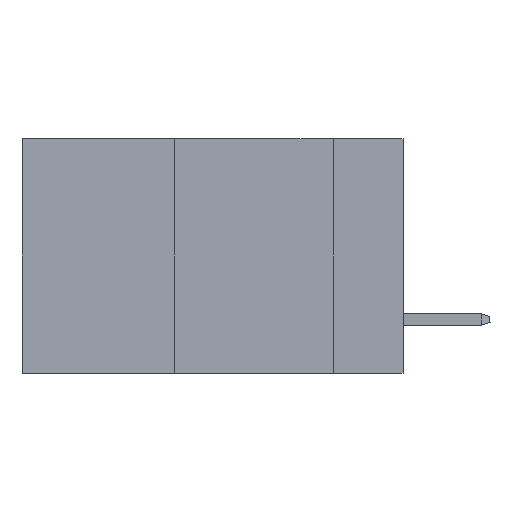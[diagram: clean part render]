
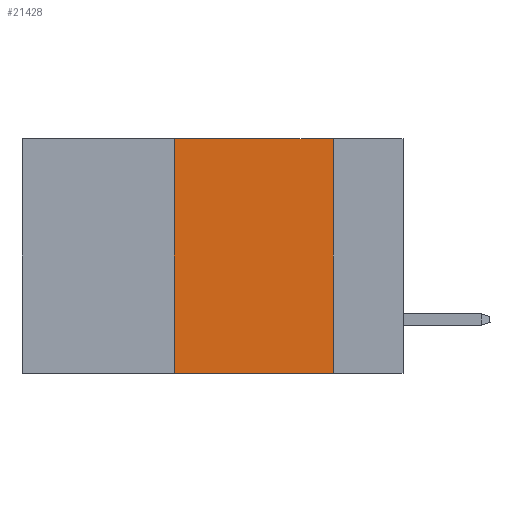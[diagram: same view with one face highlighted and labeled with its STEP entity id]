
A CAD part, left-side view. The second image highlights one B-rep face of the part: STEP entity #21428.
In plain terms, the highlighted planar face has unit normal (-1, 0, 0).
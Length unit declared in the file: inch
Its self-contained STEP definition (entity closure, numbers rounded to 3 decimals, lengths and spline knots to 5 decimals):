
#226 = CARTESIAN_POINT ( 'NONE',  ( 0., 0.11, -0.37 ) ) ;
#608 = VECTOR ( 'NONE', #22366, 39.37008 ) ;
#1459 = DIRECTION ( 'NONE',  ( 0., 0., -1. ) ) ;
#1627 = VECTOR ( 'NONE', #17815, 39.37008 ) ;
#2300 = DIRECTION ( 'NONE',  ( 0., 0., -1. ) ) ;
#2961 = CARTESIAN_POINT ( 'NONE',  ( 0., 0.11, 0. ) ) ;
#3543 = EDGE_CURVE ( 'NONE', #16228, #36907, #26728, .T. ) ;
#8606 = VERTEX_POINT ( 'NONE', #15901 ) ;
#11014 = EDGE_CURVE ( 'NONE', #8606, #16228, #23114, .T. ) ;
#11662 = DIRECTION ( 'NONE',  ( 0., -1., 0. ) ) ;
#12409 = EDGE_LOOP ( 'NONE', ( #28049, #28809, #15225, #15103 ) ) ;
#13007 = CARTESIAN_POINT ( 'NONE',  ( 0., 0.11, 0. ) ) ;
#13609 = CARTESIAN_POINT ( 'NONE',  ( 0., 0.36, 0. ) ) ;
#15103 = ORIENTED_EDGE ( 'NONE', *, *, #16697, .T. ) ;
#15225 = ORIENTED_EDGE ( 'NONE', *, *, #11014, .F. ) ;
#15299 = LINE ( 'NONE', #13007, #22468 ) ;
#15901 = CARTESIAN_POINT ( 'NONE',  ( 0., 0.36, -0.37 ) ) ;
#15935 = AXIS2_PLACEMENT_3D ( 'NONE', #28811, #28428, #2300 ) ;
#16228 = VERTEX_POINT ( 'NONE', #13609 ) ;
#16697 = EDGE_CURVE ( 'NONE', #8606, #28539, #25513, .T. ) ;
#17292 = FACE_OUTER_BOUND ( 'NONE', #12409, .T. ) ;
#17815 = DIRECTION ( 'NONE',  ( 0., 0., 1. ) ) ;
#21428 = ADVANCED_FACE ( 'NONE', ( #17292 ), #34653, .F. ) ;
#22366 = DIRECTION ( 'NONE',  ( 0., -1., 0. ) ) ;
#22468 = VECTOR ( 'NONE', #1459, 39.37008 ) ;
#23114 = LINE ( 'NONE', #34805, #1627 ) ;
#23890 = EDGE_CURVE ( 'NONE', #36907, #28539, #15299, .T. ) ;
#25513 = LINE ( 'NONE', #37398, #26067 ) ;
#26067 = VECTOR ( 'NONE', #11662, 39.37008 ) ;
#26728 = LINE ( 'NONE', #30686, #608 ) ;
#28049 = ORIENTED_EDGE ( 'NONE', *, *, #23890, .F. ) ;
#28428 = DIRECTION ( 'NONE',  ( 1., 0., 0. ) ) ;
#28539 = VERTEX_POINT ( 'NONE', #226 ) ;
#28809 = ORIENTED_EDGE ( 'NONE', *, *, #3543, .F. ) ;
#28811 = CARTESIAN_POINT ( 'NONE',  ( 0., 0.6, 0. ) ) ;
#30686 = CARTESIAN_POINT ( 'NONE',  ( 0., 0.6, 0. ) ) ;
#34653 = PLANE ( 'NONE',  #15935 ) ;
#34805 = CARTESIAN_POINT ( 'NONE',  ( 0., 0.36, 0. ) ) ;
#36907 = VERTEX_POINT ( 'NONE', #2961 ) ;
#37398 = CARTESIAN_POINT ( 'NONE',  ( 0., 0.6, -0.37 ) ) ;
